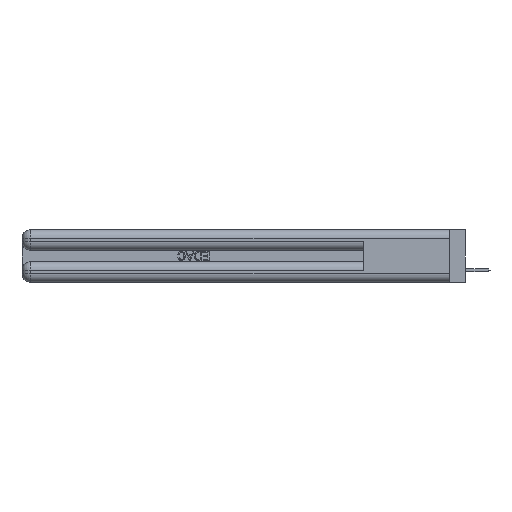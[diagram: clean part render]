
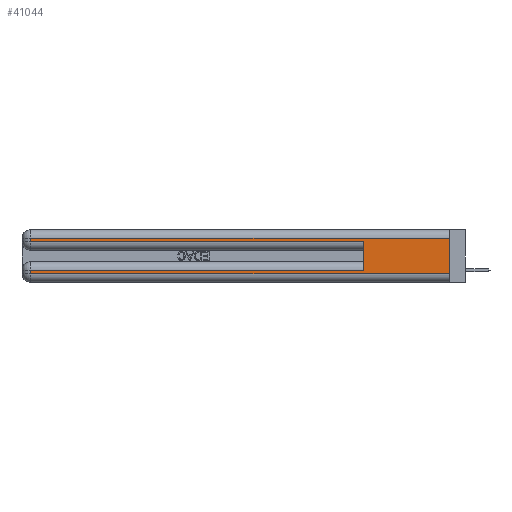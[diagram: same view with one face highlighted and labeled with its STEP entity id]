
A CAD part, left-side view. The second image highlights one B-rep face of the part: STEP entity #41044.
In plain terms, the highlighted planar face has unit normal (-1, 0, 0).
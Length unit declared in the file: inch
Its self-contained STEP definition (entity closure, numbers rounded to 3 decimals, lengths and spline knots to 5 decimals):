
#146 = DIRECTION ( 'NONE',  ( 0., 0., -1. ) ) ;
#628 = VERTEX_POINT ( 'NONE', #33190 ) ;
#696 = VECTOR ( 'NONE', #16876, 39.37008 ) ;
#964 = DIRECTION ( 'NONE',  ( 0., 0., -1. ) ) ;
#1148 = EDGE_LOOP ( 'NONE', ( #30712, #37907, #13528, #34308, #6802, #38264, #14582, #18479 ) ) ;
#3534 = CARTESIAN_POINT ( 'NONE',  ( 0., 2.94, 0.285 ) ) ;
#5281 = CARTESIAN_POINT ( 'NONE',  ( 0., 0., 0.31 ) ) ;
#5927 = CARTESIAN_POINT ( 'NONE',  ( 0., 0., 0.06 ) ) ;
#6802 = ORIENTED_EDGE ( 'NONE', *, *, #31255, .F. ) ;
#6950 = CARTESIAN_POINT ( 'NONE',  ( 0., 0., 0.37 ) ) ;
#7229 = CARTESIAN_POINT ( 'NONE',  ( 0., 2.94, 0.37 ) ) ;
#7279 = CARTESIAN_POINT ( 'NONE',  ( 0., 2.94, 0.085 ) ) ;
#8096 = EDGE_CURVE ( 'NONE', #25869, #42349, #12111, .T. ) ;
#8204 = CARTESIAN_POINT ( 'NONE',  ( 0., 2.94, 0.06 ) ) ;
#9485 = FACE_OUTER_BOUND ( 'NONE', #1148, .T. ) ;
#9731 = LINE ( 'NONE', #37151, #696 ) ;
#11304 = DIRECTION ( 'NONE',  ( 0., 1., 0. ) ) ;
#12111 = LINE ( 'NONE', #23458, #42270 ) ;
#13528 = ORIENTED_EDGE ( 'NONE', *, *, #17935, .T. ) ;
#14090 = DIRECTION ( 'NONE',  ( 0., -1., 0. ) ) ;
#14582 = ORIENTED_EDGE ( 'NONE', *, *, #8096, .T. ) ;
#15693 = LINE ( 'NONE', #6950, #33741 ) ;
#16526 = LINE ( 'NONE', #7229, #37703 ) ;
#16876 = DIRECTION ( 'NONE',  ( 0., -1., 0. ) ) ;
#17124 = VECTOR ( 'NONE', #25207, 39.37008 ) ;
#17935 = EDGE_CURVE ( 'NONE', #31159, #29930, #16526, .T. ) ;
#17958 = DIRECTION ( 'NONE',  ( 0., 0., 1. ) ) ;
#18024 = VECTOR ( 'NONE', #17958, 39.37008 ) ;
#18479 = ORIENTED_EDGE ( 'NONE', *, *, #34313, .T. ) ;
#19754 = LINE ( 'NONE', #31411, #17124 ) ;
#20127 = LINE ( 'NONE', #37650, #32923 ) ;
#21732 = EDGE_CURVE ( 'NONE', #41922, #31159, #31904, .T. ) ;
#22901 = VECTOR ( 'NONE', #11304, 39.37008 ) ;
#23458 = CARTESIAN_POINT ( 'NONE',  ( 0., 2.94, 0.37 ) ) ;
#24590 = EDGE_CURVE ( 'NONE', #41922, #43295, #15693, .T. ) ;
#25166 = CARTESIAN_POINT ( 'NONE',  ( 0., 0., 0.37 ) ) ;
#25207 = DIRECTION ( 'NONE',  ( 0., 1., 0. ) ) ;
#25315 = DIRECTION ( 'NONE',  ( 1., 0., 0. ) ) ;
#25869 = VERTEX_POINT ( 'NONE', #7279 ) ;
#27080 = LINE ( 'NONE', #31181, #18024 ) ;
#28552 = EDGE_CURVE ( 'NONE', #29930, #628, #9731, .T. ) ;
#29930 = VERTEX_POINT ( 'NONE', #3534 ) ;
#30712 = ORIENTED_EDGE ( 'NONE', *, *, #24590, .F. ) ;
#30974 = DIRECTION ( 'NONE',  ( 0., 0., -1. ) ) ;
#31159 = VERTEX_POINT ( 'NONE', #34005 ) ;
#31181 = CARTESIAN_POINT ( 'NONE',  ( 0., 0.6, 0.145 ) ) ;
#31255 = EDGE_CURVE ( 'NONE', #42281, #628, #27080, .T. ) ;
#31411 = CARTESIAN_POINT ( 'NONE',  ( 0., 0., 0.085 ) ) ;
#31815 = PLANE ( 'NONE',  #36225 ) ;
#31904 = LINE ( 'NONE', #42056, #22901 ) ;
#32923 = VECTOR ( 'NONE', #14090, 39.37008 ) ;
#33190 = CARTESIAN_POINT ( 'NONE',  ( 0., 0.6, 0.285 ) ) ;
#33741 = VECTOR ( 'NONE', #37036, 39.37008 ) ;
#34005 = CARTESIAN_POINT ( 'NONE',  ( 0., 2.94, 0.31 ) ) ;
#34308 = ORIENTED_EDGE ( 'NONE', *, *, #28552, .T. ) ;
#34313 = EDGE_CURVE ( 'NONE', #42349, #43295, #20127, .T. ) ;
#36225 = AXIS2_PLACEMENT_3D ( 'NONE', #25166, #25315, #964 ) ;
#37036 = DIRECTION ( 'NONE',  ( 0., 0., -1. ) ) ;
#37151 = CARTESIAN_POINT ( 'NONE',  ( 0., 0., 0.285 ) ) ;
#37650 = CARTESIAN_POINT ( 'NONE',  ( 0., 0., 0.06 ) ) ;
#37703 = VECTOR ( 'NONE', #30974, 39.37008 ) ;
#37817 = CARTESIAN_POINT ( 'NONE',  ( 0., 0.6, 0.085 ) ) ;
#37907 = ORIENTED_EDGE ( 'NONE', *, *, #21732, .T. ) ;
#38264 = ORIENTED_EDGE ( 'NONE', *, *, #38358, .T. ) ;
#38358 = EDGE_CURVE ( 'NONE', #42281, #25869, #19754, .T. ) ;
#41044 = ADVANCED_FACE ( 'NONE', ( #9485 ), #31815, .F. ) ;
#41922 = VERTEX_POINT ( 'NONE', #5281 ) ;
#42056 = CARTESIAN_POINT ( 'NONE',  ( 0., 0., 0.31 ) ) ;
#42270 = VECTOR ( 'NONE', #146, 39.37008 ) ;
#42281 = VERTEX_POINT ( 'NONE', #37817 ) ;
#42349 = VERTEX_POINT ( 'NONE', #8204 ) ;
#43295 = VERTEX_POINT ( 'NONE', #5927 ) ;
